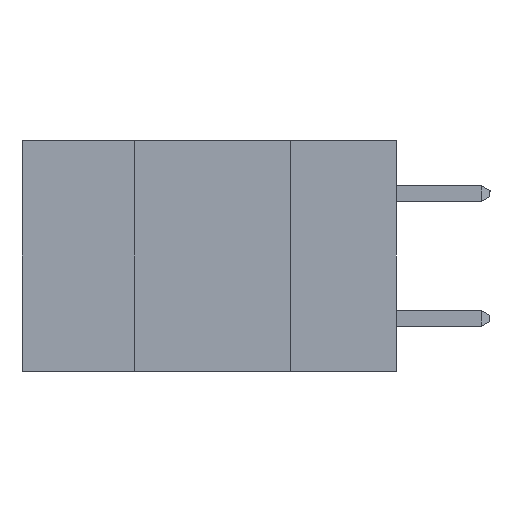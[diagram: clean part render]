
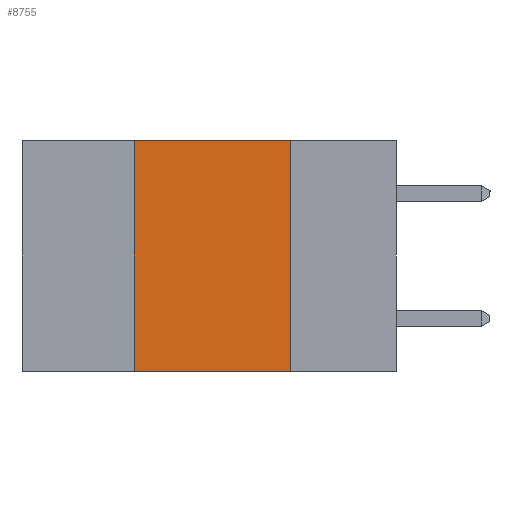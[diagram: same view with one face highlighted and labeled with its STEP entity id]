
A CAD part, left-side view. The second image highlights one B-rep face of the part: STEP entity #8755.
In plain terms, the highlighted planar face has unit normal (-1, 0, 0).
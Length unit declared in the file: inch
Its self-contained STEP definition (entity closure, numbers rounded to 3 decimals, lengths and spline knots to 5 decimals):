
#31 = CARTESIAN_POINT ( 'NONE',  ( 0., 0.42, -0.37 ) ) ;
#453 = EDGE_CURVE ( 'NONE', #4596, #11865, #12317, .T. ) ;
#805 = AXIS2_PLACEMENT_3D ( 'NONE', #10110, #9909, #3771 ) ;
#924 = CARTESIAN_POINT ( 'NONE',  ( 0., 0.17, -0.37 ) ) ;
#1269 = VECTOR ( 'NONE', #1642, 39.37008 ) ;
#1603 = DIRECTION ( 'NONE',  ( 0., -1., 0. ) ) ;
#1642 = DIRECTION ( 'NONE',  ( 0., -1., 0. ) ) ;
#1868 = CARTESIAN_POINT ( 'NONE',  ( 0., 0.6, 0. ) ) ;
#2125 = ORIENTED_EDGE ( 'NONE', *, *, #5782, .F. ) ;
#2932 = CARTESIAN_POINT ( 'NONE',  ( 0., 0.6, -0.37 ) ) ;
#3118 = EDGE_LOOP ( 'NONE', ( #3234, #2125, #11134, #13076 ) ) ;
#3134 = VECTOR ( 'NONE', #1603, 39.37008 ) ;
#3234 = ORIENTED_EDGE ( 'NONE', *, *, #4951, .F. ) ;
#3646 = FACE_OUTER_BOUND ( 'NONE', #3118, .T. ) ;
#3771 = DIRECTION ( 'NONE',  ( 0., 0., -1. ) ) ;
#4281 = CARTESIAN_POINT ( 'NONE',  ( 0., 0.17, -0.37 ) ) ;
#4417 = CARTESIAN_POINT ( 'NONE',  ( 0., 0.17, 0. ) ) ;
#4596 = VERTEX_POINT ( 'NONE', #31 ) ;
#4951 = EDGE_CURVE ( 'NONE', #8995, #10920, #12665, .T. ) ;
#4982 = CARTESIAN_POINT ( 'NONE',  ( 0., 0.42, 0. ) ) ;
#5782 = EDGE_CURVE ( 'NONE', #11865, #8995, #8891, .T. ) ;
#8552 = VECTOR ( 'NONE', #12599, 39.37008 ) ;
#8755 = ADVANCED_FACE ( 'NONE', ( #3646 ), #12236, .F. ) ;
#8891 = LINE ( 'NONE', #1868, #3134 ) ;
#8995 = VERTEX_POINT ( 'NONE', #4417 ) ;
#9909 = DIRECTION ( 'NONE',  ( 1., 0., 0. ) ) ;
#10110 = CARTESIAN_POINT ( 'NONE',  ( 0., 0.6, 0. ) ) ;
#10437 = EDGE_CURVE ( 'NONE', #4596, #10920, #11177, .T. ) ;
#10920 = VERTEX_POINT ( 'NONE', #924 ) ;
#11134 = ORIENTED_EDGE ( 'NONE', *, *, #453, .F. ) ;
#11177 = LINE ( 'NONE', #2932, #1269 ) ;
#11865 = VERTEX_POINT ( 'NONE', #4982 ) ;
#12236 = PLANE ( 'NONE',  #805 ) ;
#12317 = LINE ( 'NONE', #13339, #12334 ) ;
#12334 = VECTOR ( 'NONE', #12449, 39.37008 ) ;
#12449 = DIRECTION ( 'NONE',  ( 0., 0., 1. ) ) ;
#12599 = DIRECTION ( 'NONE',  ( 0., 0., -1. ) ) ;
#12665 = LINE ( 'NONE', #4281, #8552 ) ;
#13076 = ORIENTED_EDGE ( 'NONE', *, *, #10437, .T. ) ;
#13339 = CARTESIAN_POINT ( 'NONE',  ( 0., 0.42, -0.37 ) ) ;
